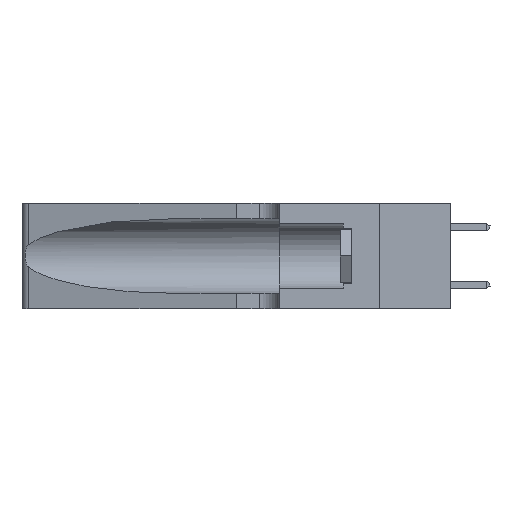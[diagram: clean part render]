
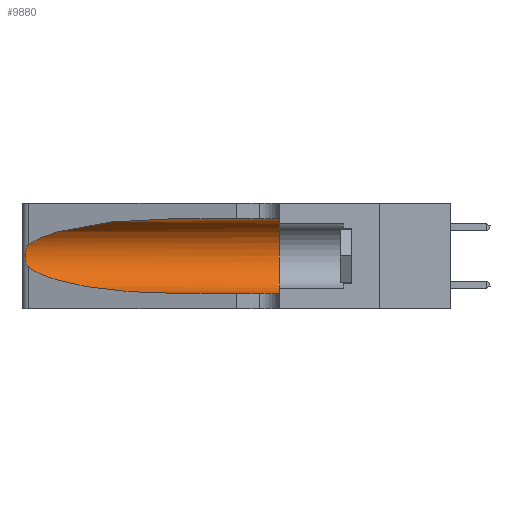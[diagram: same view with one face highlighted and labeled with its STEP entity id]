
A CAD part, left-side view. The second image highlights one B-rep face of the part: STEP entity #9880.
In plain terms, the highlighted cylindrical face has radius 3.308 mm (diameter 6.617 mm), a partial arc.
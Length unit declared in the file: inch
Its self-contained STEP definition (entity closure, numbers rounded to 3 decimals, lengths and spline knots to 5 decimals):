
#436 = LINE ( 'NONE', #7149, #15909 ) ;
#879 = CIRCLE ( 'NONE', #23154, 0.13025 ) ;
#1248 = CARTESIAN_POINT ( 'NONE',  ( 0.25555, 1.22994, 0.2215 ) ) ;
#1279 = EDGE_CURVE ( 'NONE', #37251, #6449, #29435, .T. ) ;
#1379 = CARTESIAN_POINT ( 'NONE',  ( 0.25854, 1.2359, 0.20912 ) ) ;
#1556 = CARTESIAN_POINT ( 'NONE',  ( 0.2373, 1.15595, 0.08982 ) ) ;
#3942 = ORIENTED_EDGE ( 'NONE', *, *, #22711, .T. ) ;
#4386 = CARTESIAN_POINT ( 'NONE',  ( 0.25487, 1.22718, 0.22369 ) ) ;
#4533 = CARTESIAN_POINT ( 'NONE',  ( 0.26075, 1.23896, 0.19203 ) ) ;
#4713 = CARTESIAN_POINT ( 'NONE',  ( 0.25487, 1.22718, 0.14631 ) ) ;
#4875 = CYLINDRICAL_SURFACE ( 'NONE', #8916, 0.13025 ) ;
#5077 = CARTESIAN_POINT ( 'NONE',  ( 0.25487, 1.22718, 0.22369 ) ) ;
#5407 = DIRECTION ( 'NONE',  ( 0., -1., 0. ) ) ;
#6449 = VERTEX_POINT ( 'NONE', #18832 ) ;
#7149 = CARTESIAN_POINT ( 'NONE',  ( 0.1305, 1.61858, 0.31525 ) ) ;
#7644 = CARTESIAN_POINT ( 'NONE',  ( 0.1305, 1.61858, 0.05475 ) ) ;
#7659 = CARTESIAN_POINT ( 'NONE',  ( 0.26017, 1.23833, 0.17102 ) ) ;
#7954 = CARTESIAN_POINT ( 'NONE',  ( 0.1305, 0.35, 0.185 ) ) ;
#8916 = AXIS2_PLACEMENT_3D ( 'NONE', #9297, #36836, #27777 ) ;
#9297 = CARTESIAN_POINT ( 'NONE',  ( 0.1305, 1.61858, 0.185 ) ) ;
#9880 = ADVANCED_FACE ( 'NONE', ( #29433 ), #4875, .F. ) ;
#10245 = DIRECTION ( 'NONE',  ( 0., -1., 0. ) ) ;
#10566 = CARTESIAN_POINT ( 'NONE',  ( 0.1305, 0.35, 0.31525 ) ) ;
#10748 = CARTESIAN_POINT ( 'NONE',  ( 0.25789, 1.23486, 0.15765 ) ) ;
#10924 = EDGE_CURVE ( 'NONE', #29234, #6449, #879, .T. ) ;
#11039 = DIRECTION ( 'NONE',  ( 0., 0., 1. ) ) ;
#12332 = EDGE_LOOP ( 'NONE', ( #37898, #3942, #36333, #34375, #21712, #13150 ) ) ;
#12976 = EDGE_CURVE ( 'NONE', #25319, #28311, #28567, .T. ) ;
#13150 = ORIENTED_EDGE ( 'NONE', *, *, #22061, .F. ) ;
#13794 = CARTESIAN_POINT ( 'NONE',  ( 0.25555, 1.22993, 0.14849 ) ) ;
#15909 = VECTOR ( 'NONE', #10245, 39.37008 ) ;
#16647 = CARTESIAN_POINT ( 'NONE',  ( 0.25487, 1.22718, 0.22369 ) ) ;
#16828 = B_SPLINE_CURVE_WITH_KNOTS ( 'NONE', 3,
 ( #4386, #1248, #38127, #19885, #1379, #23003, #4533, #26129, #7659, #29165, #10748, #32209, #13794, #35226 ),
 .UNSPECIFIED., .F., .F.,
 ( 4, 2, 2, 2, 2, 2, 4 ),
 ( 0., 0.00027, 0.00053, 0.00107, 0.0016, 0.00187, 0.00214 ),
 .UNSPECIFIED. ) ;
#17869 = CARTESIAN_POINT ( 'NONE',  ( 0.25487, 1.22718, 0.14631 ) ) ;
#18832 = CARTESIAN_POINT ( 'NONE',  ( 0.1305, 0.35, 0.05475 ) ) ;
#19885 = CARTESIAN_POINT ( 'NONE',  ( 0.25787, 1.23484, 0.2124 ) ) ;
#20056 = CARTESIAN_POINT ( 'NONE',  ( 0.18966, 0.96281, 0.05475 ) ) ;
#20089 = EDGE_CURVE ( 'NONE', #32111, #37251, #38930, .T. ) ;
#21258 = VECTOR ( 'NONE', #5407, 39.37008 ) ;
#21712 = ORIENTED_EDGE ( 'NONE', *, *, #10924, .F. ) ;
#22061 = EDGE_CURVE ( 'NONE', #25319, #29234, #436, .T. ) ;
#22711 = EDGE_CURVE ( 'NONE', #28311, #32111, #16828, .T. ) ;
#23003 = CARTESIAN_POINT ( 'NONE',  ( 0.26018, 1.23835, 0.19895 ) ) ;
#23154 = AXIS2_PLACEMENT_3D ( 'NONE', #7954, #29459, #11039 ) ;
#23556 = CARTESIAN_POINT ( 'NONE',  ( 0.2373, 1.15595, 0.28018 ) ) ;
#25319 = VERTEX_POINT ( 'NONE', #34439 ) ;
#26129 = CARTESIAN_POINT ( 'NONE',  ( 0.26075, 1.23896, 0.178 ) ) ;
#26309 = CARTESIAN_POINT ( 'NONE',  ( 0.1305, 0.72297, 0.05475 ) ) ;
#26542 = CARTESIAN_POINT ( 'NONE',  ( 0.1305, 0.72297, 0.05475 ) ) ;
#27777 = DIRECTION ( 'NONE',  ( 0., 0., -1. ) ) ;
#28311 = VERTEX_POINT ( 'NONE', #16647 ) ;
#28567 =( BOUNDED_CURVE ( )  B_SPLINE_CURVE ( 3, ( #35610, #38637, #23556, #5077 ),
 .UNSPECIFIED., .F., .T. ) 
 B_SPLINE_CURVE_WITH_KNOTS ( ( 4, 4 ),
 ( 1.5708, 2.84003 ),
 .UNSPECIFIED. ) 
 CURVE ( )  GEOMETRIC_REPRESENTATION_ITEM ( )  RATIONAL_B_SPLINE_CURVE ( ( 1., 0.87, 0.87, 1. ) ) 
 REPRESENTATION_ITEM ( '' )  );
#29165 = CARTESIAN_POINT ( 'NONE',  ( 0.25856, 1.23593, 0.16098 ) ) ;
#29234 = VERTEX_POINT ( 'NONE', #10566 ) ;
#29433 = FACE_OUTER_BOUND ( 'NONE', #12332, .T. ) ;
#29435 = LINE ( 'NONE', #7644, #21258 ) ;
#29459 = DIRECTION ( 'NONE',  ( 0., 1., 0. ) ) ;
#32111 = VERTEX_POINT ( 'NONE', #17869 ) ;
#32209 = CARTESIAN_POINT ( 'NONE',  ( 0.25639, 1.23186, 0.15144 ) ) ;
#34375 = ORIENTED_EDGE ( 'NONE', *, *, #1279, .T. ) ;
#34439 = CARTESIAN_POINT ( 'NONE',  ( 0.1305, 0.72297, 0.31525 ) ) ;
#35226 = CARTESIAN_POINT ( 'NONE',  ( 0.25487, 1.22718, 0.14631 ) ) ;
#35610 = CARTESIAN_POINT ( 'NONE',  ( 0.1305, 0.72297, 0.31525 ) ) ;
#36333 = ORIENTED_EDGE ( 'NONE', *, *, #20089, .T. ) ;
#36836 = DIRECTION ( 'NONE',  ( 0., -1., 0. ) ) ;
#37251 = VERTEX_POINT ( 'NONE', #26542 ) ;
#37898 = ORIENTED_EDGE ( 'NONE', *, *, #12976, .T. ) ;
#38127 = CARTESIAN_POINT ( 'NONE',  ( 0.25639, 1.23184, 0.21858 ) ) ;
#38637 = CARTESIAN_POINT ( 'NONE',  ( 0.18966, 0.96281, 0.31525 ) ) ;
#38930 =( BOUNDED_CURVE ( )  B_SPLINE_CURVE ( 3, ( #4713, #1556, #20056, #26309 ),
 .UNSPECIFIED., .F., .T. ) 
 B_SPLINE_CURVE_WITH_KNOTS ( ( 4, 4 ),
 ( 3.44316, 4.71239 ),
 .UNSPECIFIED. ) 
 CURVE ( )  GEOMETRIC_REPRESENTATION_ITEM ( )  RATIONAL_B_SPLINE_CURVE ( ( 1., 0.87, 0.87, 1. ) ) 
 REPRESENTATION_ITEM ( '' )  );
